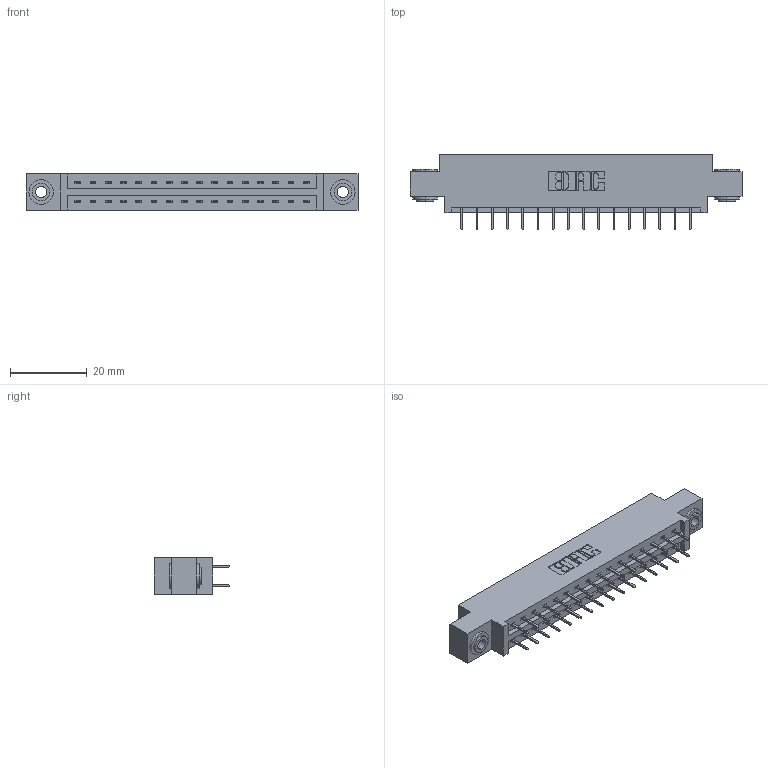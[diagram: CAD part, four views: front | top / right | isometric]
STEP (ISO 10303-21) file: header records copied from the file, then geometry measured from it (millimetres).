
FILE_DESCRIPTION (( 'STEP AP203' ), '1' );
FILE_NAME ('387-032-524-803.STEP', '2019-10-17T15:42:43', ( '' ), ( '' ), 'SwSTEP 2.0', 'SolidWorks 2016', '' );
FILE_SCHEMA (( 'CONFIG_CONTROL_DESIGN' ));
Length unit declared in the file: inch
Products named in the file (4): 345-250-002_345-250-002-102; 345-292-001_345-293-124; 337 Part_0.170 Offset - 0.156 Dia-TH; 387-032-524-803
Assembly tree (35 placements, depth 2):
  387-032-524-803
    337 Part_0.170 Offset - 0.156 Dia-TH
    345-292-001_345-293-124  x32
    345-250-002_345-250-002-102  x2
Bounding box: 86.41 x 19.69 x 9.4 mm (x, y, z)
Volume: 8614 mm3; surface area: 9667.9 mm2
Topology: 35 solids, 35 shells, 2012 faces, 5679 edges, 3654 vertices
Faces by surface type: plane 1492, cylinder 512, cone 8
Entity records: 16624 total; most frequent: CARTESIAN_POINT 2797, ORIENTED_EDGE 2726, DIRECTION 2461, EDGE_CURVE 1363, VECTOR 1215, LINE 1215, VERTEX_POINT 902, AXIS2_PLACEMENT_3D 623
